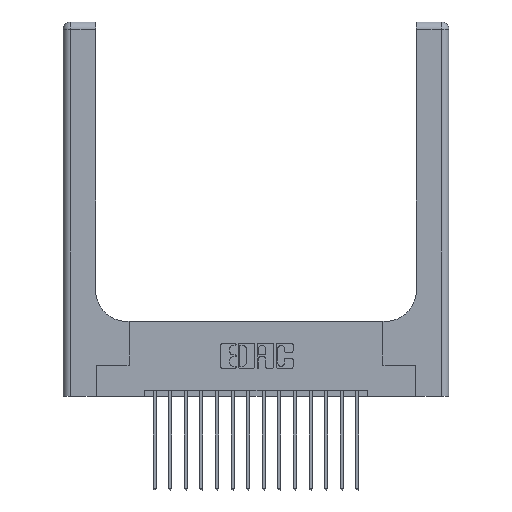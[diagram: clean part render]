
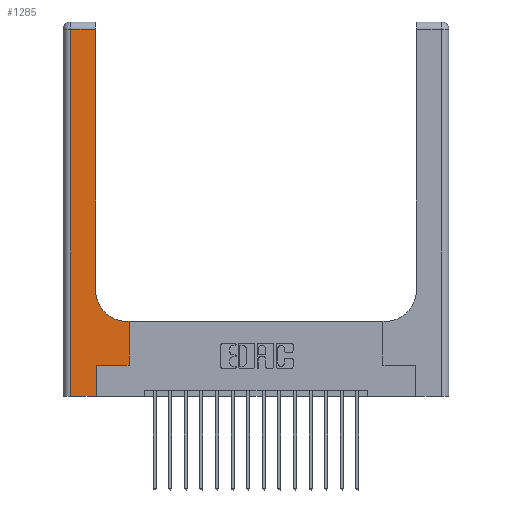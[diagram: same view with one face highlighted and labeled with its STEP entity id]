
A CAD part, top view. The second image highlights one B-rep face of the part: STEP entity #1285.
In plain terms, the highlighted planar face has unit normal (0, 0, 1).
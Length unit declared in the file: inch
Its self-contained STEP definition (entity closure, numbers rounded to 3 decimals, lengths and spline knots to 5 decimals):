
#1 = ORIENTED_EDGE ( 'NONE', *, *, #374, .T. ) ;
#245 = VECTOR ( 'NONE', #10932, 39.37008 ) ;
#374 = EDGE_CURVE ( 'NONE', #2850, #13027, #12959, .T. ) ;
#404 = VECTOR ( 'NONE', #1454, 39.37008 ) ;
#443 = EDGE_LOOP ( 'NONE', ( #2459, #3343, #1, #10607, #5554, #1988, #8039, #1210, #9788 ) ) ;
#681 = CARTESIAN_POINT ( 'NONE',  ( 0., 3., 0.37 ) ) ;
#1131 = EDGE_CURVE ( 'NONE', #16245, #15562, #17929, .T. ) ;
#1210 = ORIENTED_EDGE ( 'NONE', *, *, #12292, .T. ) ;
#1215 = VERTEX_POINT ( 'NONE', #8746 ) ;
#1285 = ADVANCED_FACE ( 'NONE', ( #1934 ), #6639, .F. ) ;
#1405 = CARTESIAN_POINT ( 'NONE',  ( 0.528, 0.25, 0.37 ) ) ;
#1454 = DIRECTION ( 'NONE',  ( -1., 0., 0. ) ) ;
#1901 = AXIS2_PLACEMENT_3D ( 'NONE', #2381, #11141, #5330 ) ;
#1934 = FACE_OUTER_BOUND ( 'NONE', #443, .T. ) ;
#1988 = ORIENTED_EDGE ( 'NONE', *, *, #10997, .T. ) ;
#2004 = CIRCLE ( 'NONE', #1901, 0.25 ) ;
#2060 = CARTESIAN_POINT ( 'NONE',  ( 0., 0., 0.37 ) ) ;
#2381 = CARTESIAN_POINT ( 'NONE',  ( 0.51, 0.85, 0.37 ) ) ;
#2459 = ORIENTED_EDGE ( 'NONE', *, *, #11343, .T. ) ;
#2850 = VERTEX_POINT ( 'NONE', #12367 ) ;
#3343 = ORIENTED_EDGE ( 'NONE', *, *, #16986, .T. ) ;
#3426 = DIRECTION ( 'NONE',  ( 0., 0., -1. ) ) ;
#3934 = VERTEX_POINT ( 'NONE', #14322 ) ;
#4221 = CARTESIAN_POINT ( 'NONE',  ( 0., 2.94, 0.37 ) ) ;
#5110 = DIRECTION ( 'NONE',  ( 1., 0., 0. ) ) ;
#5147 = VECTOR ( 'NONE', #11077, 39.37008 ) ;
#5178 = DIRECTION ( 'NONE',  ( 0., 1., 0. ) ) ;
#5330 = DIRECTION ( 'NONE',  ( 1., 0., 0. ) ) ;
#5554 = ORIENTED_EDGE ( 'NONE', *, *, #9701, .T. ) ;
#5731 = DIRECTION ( 'NONE',  ( 0., -1., 0. ) ) ;
#5892 = VECTOR ( 'NONE', #5178, 39.37008 ) ;
#6112 = CARTESIAN_POINT ( 'NONE',  ( 0.265, 0., 0.37 ) ) ;
#6320 = LINE ( 'NONE', #10844, #16183 ) ;
#6439 = DIRECTION ( 'NONE',  ( 1., 0., 0. ) ) ;
#6639 = PLANE ( 'NONE',  #8038 ) ;
#6739 = CARTESIAN_POINT ( 'NONE',  ( 0.26, 0.6, 0.37 ) ) ;
#7349 = VERTEX_POINT ( 'NONE', #6112 ) ;
#8038 = AXIS2_PLACEMENT_3D ( 'NONE', #681, #3426, #9519 ) ;
#8039 = ORIENTED_EDGE ( 'NONE', *, *, #1131, .T. ) ;
#8746 = CARTESIAN_POINT ( 'NONE',  ( 0.26, 2.94, 0.37 ) ) ;
#9373 = CARTESIAN_POINT ( 'NONE',  ( 0.06, 0., 0.37 ) ) ;
#9519 = DIRECTION ( 'NONE',  ( -1., 0., 0. ) ) ;
#9701 = EDGE_CURVE ( 'NONE', #7349, #3934, #13485, .T. ) ;
#9729 = EDGE_CURVE ( 'NONE', #13027, #7349, #13357, .T. ) ;
#9788 = ORIENTED_EDGE ( 'NONE', *, *, #10712, .T. ) ;
#10607 = ORIENTED_EDGE ( 'NONE', *, *, #9729, .T. ) ;
#10712 = EDGE_CURVE ( 'NONE', #13109, #18329, #2004, .T. ) ;
#10844 = CARTESIAN_POINT ( 'NONE',  ( 0.26, 3., 0.37 ) ) ;
#10932 = DIRECTION ( 'NONE',  ( 0., 1., 0. ) ) ;
#10963 = CARTESIAN_POINT ( 'NONE',  ( 0.265, 0.25, 0.37 ) ) ;
#10997 = EDGE_CURVE ( 'NONE', #3934, #16245, #13679, .T. ) ;
#11077 = DIRECTION ( 'NONE',  ( -1., 0., 0. ) ) ;
#11141 = DIRECTION ( 'NONE',  ( 0., 0., -1. ) ) ;
#11343 = EDGE_CURVE ( 'NONE', #18329, #1215, #6320, .T. ) ;
#12292 = EDGE_CURVE ( 'NONE', #15562, #13109, #14061, .T. ) ;
#12367 = CARTESIAN_POINT ( 'NONE',  ( 0.06, 2.94, 0.37 ) ) ;
#12771 = LINE ( 'NONE', #4221, #404 ) ;
#12959 = LINE ( 'NONE', #13049, #17513 ) ;
#13027 = VERTEX_POINT ( 'NONE', #9373 ) ;
#13049 = CARTESIAN_POINT ( 'NONE',  ( 0.06, 3., 0.37 ) ) ;
#13109 = VERTEX_POINT ( 'NONE', #15479 ) ;
#13357 = LINE ( 'NONE', #2060, #16446 ) ;
#13485 = LINE ( 'NONE', #14992, #245 ) ;
#13675 = CARTESIAN_POINT ( 'NONE',  ( 0.528, 0.6, 0.37 ) ) ;
#13679 = LINE ( 'NONE', #10963, #15000 ) ;
#13850 = CARTESIAN_POINT ( 'NONE',  ( 0.26, 0.85, 0.37 ) ) ;
#14061 = LINE ( 'NONE', #6739, #5147 ) ;
#14322 = CARTESIAN_POINT ( 'NONE',  ( 0.265, 0.25, 0.37 ) ) ;
#14992 = CARTESIAN_POINT ( 'NONE',  ( 0.265, 0., 0.37 ) ) ;
#15000 = VECTOR ( 'NONE', #6439, 39.37008 ) ;
#15479 = CARTESIAN_POINT ( 'NONE',  ( 0.51, 0.6, 0.37 ) ) ;
#15562 = VERTEX_POINT ( 'NONE', #13675 ) ;
#16183 = VECTOR ( 'NONE', #16894, 39.37008 ) ;
#16245 = VERTEX_POINT ( 'NONE', #1405 ) ;
#16446 = VECTOR ( 'NONE', #5110, 39.37008 ) ;
#16894 = DIRECTION ( 'NONE',  ( 0., 1., 0. ) ) ;
#16986 = EDGE_CURVE ( 'NONE', #1215, #2850, #12771, .T. ) ;
#17513 = VECTOR ( 'NONE', #5731, 39.37008 ) ;
#17929 = LINE ( 'NONE', #18023, #5892 ) ;
#18023 = CARTESIAN_POINT ( 'NONE',  ( 0.528, 0.25, 0.37 ) ) ;
#18329 = VERTEX_POINT ( 'NONE', #13850 ) ;
